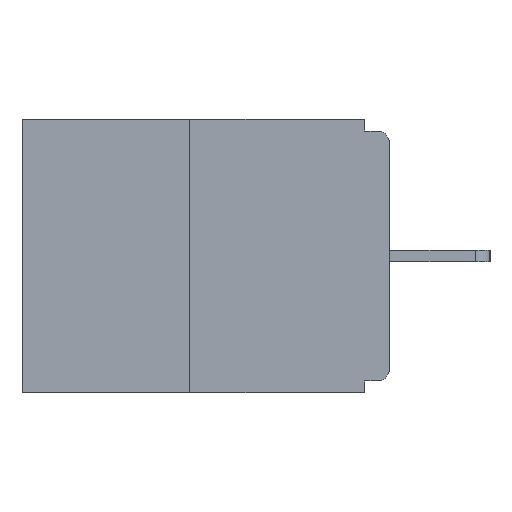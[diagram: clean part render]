
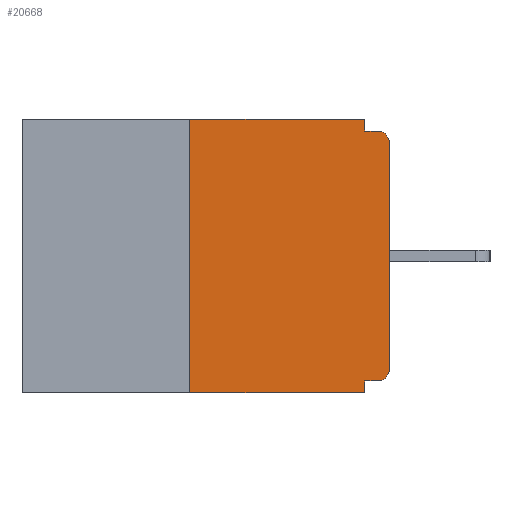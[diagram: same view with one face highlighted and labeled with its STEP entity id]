
A CAD part, left-side view. The second image highlights one B-rep face of the part: STEP entity #20668.
In plain terms, the highlighted planar face has unit normal (-1, 0, 0).
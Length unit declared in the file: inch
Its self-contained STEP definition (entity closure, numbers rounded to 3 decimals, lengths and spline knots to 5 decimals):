
#95 = EDGE_CURVE ( 'NONE', #3770, #21573, #4063, .T. ) ;
#250 = CARTESIAN_POINT ( 'NONE',  ( 0., 0.031, 0. ) ) ;
#340 = VECTOR ( 'NONE', #15545, 39.37008 ) ;
#508 = CARTESIAN_POINT ( 'NONE',  ( 0., 0.031, 0. ) ) ;
#1154 = VERTEX_POINT ( 'NONE', #3916 ) ;
#1259 = DIRECTION ( 'NONE',  ( -1., 0., 0. ) ) ;
#1460 = CARTESIAN_POINT ( 'NONE',  ( 0., 0.015, -0.328 ) ) ;
#1532 = EDGE_CURVE ( 'NONE', #21573, #20040, #19055, .T. ) ;
#1893 = DIRECTION ( 'NONE',  ( 0., -1., 0. ) ) ;
#2144 = DIRECTION ( 'NONE',  ( 0., 0., -1. ) ) ;
#2250 = ORIENTED_EDGE ( 'NONE', *, *, #19633, .T. ) ;
#2343 = CARTESIAN_POINT ( 'NONE',  ( 0., 0.25, 0. ) ) ;
#2382 = EDGE_CURVE ( 'NONE', #19402, #3770, #9972, .T. ) ;
#3080 = LINE ( 'NONE', #21644, #3811 ) ;
#3449 = LINE ( 'NONE', #3668, #11218 ) ;
#3616 = LINE ( 'NONE', #8801, #340 ) ;
#3668 = CARTESIAN_POINT ( 'NONE',  ( 0., 0.46, -0.343 ) ) ;
#3770 = VERTEX_POINT ( 'NONE', #19185 ) ;
#3811 = VECTOR ( 'NONE', #6506, 39.37008 ) ;
#3837 = LINE ( 'NONE', #508, #6637 ) ;
#3916 = CARTESIAN_POINT ( 'NONE',  ( 0., 0.031, -0.015 ) ) ;
#3955 = DIRECTION ( 'NONE',  ( 0., 0., 1. ) ) ;
#4018 = ORIENTED_EDGE ( 'NONE', *, *, #1532, .T. ) ;
#4038 = EDGE_CURVE ( 'NONE', #14052, #16730, #12008, .T. ) ;
#4063 = LINE ( 'NONE', #20645, #6922 ) ;
#4556 = ORIENTED_EDGE ( 'NONE', *, *, #2382, .T. ) ;
#5302 = AXIS2_PLACEMENT_3D ( 'NONE', #16389, #1259, #7968 ) ;
#5350 = PLANE ( 'NONE',  #6602 ) ;
#5366 = DIRECTION ( 'NONE',  ( 0., 0., 1. ) ) ;
#5571 = VECTOR ( 'NONE', #16714, 39.37008 ) ;
#5863 = VERTEX_POINT ( 'NONE', #250 ) ;
#5922 = VECTOR ( 'NONE', #5366, 39.37008 ) ;
#6506 = DIRECTION ( 'NONE',  ( 0., -1., 0. ) ) ;
#6602 = AXIS2_PLACEMENT_3D ( 'NONE', #15522, #11878, #2144 ) ;
#6626 = ORIENTED_EDGE ( 'NONE', *, *, #11526, .F. ) ;
#6637 = VECTOR ( 'NONE', #8999, 39.37008 ) ;
#6922 = VECTOR ( 'NONE', #3955, 39.37008 ) ;
#7847 = DIRECTION ( 'NONE',  ( 0., 0., -1. ) ) ;
#7968 = DIRECTION ( 'NONE',  ( 0., 0., -1. ) ) ;
#8144 = DIRECTION ( 'NONE',  ( 0., 0., -1. ) ) ;
#8559 = ORIENTED_EDGE ( 'NONE', *, *, #95, .T. ) ;
#8592 = CARTESIAN_POINT ( 'NONE',  ( 0., 0.031, -0.328 ) ) ;
#8801 = CARTESIAN_POINT ( 'NONE',  ( 0., 0., -0.328 ) ) ;
#8980 = FACE_OUTER_BOUND ( 'NONE', #16763, .T. ) ;
#8999 = DIRECTION ( 'NONE',  ( 0., 0., -1. ) ) ;
#9675 = EDGE_CURVE ( 'NONE', #1154, #20040, #3080, .T. ) ;
#9744 = EDGE_CURVE ( 'NONE', #5863, #1154, #3837, .T. ) ;
#9869 = VERTEX_POINT ( 'NONE', #12994 ) ;
#9972 = CIRCLE ( 'NONE', #19124, 0.015 ) ;
#10105 = ORIENTED_EDGE ( 'NONE', *, *, #10378, .F. ) ;
#10378 = EDGE_CURVE ( 'NONE', #13232, #9869, #21122, .T. ) ;
#10907 = CARTESIAN_POINT ( 'NONE',  ( 0., 0., -0.03 ) ) ;
#11218 = VECTOR ( 'NONE', #1893, 39.37008 ) ;
#11261 = CARTESIAN_POINT ( 'NONE',  ( 0., 0.015, -0.313 ) ) ;
#11526 = EDGE_CURVE ( 'NONE', #19402, #13232, #3616, .T. ) ;
#11878 = DIRECTION ( 'NONE',  ( 1., 0., 0. ) ) ;
#12008 = LINE ( 'NONE', #18848, #5922 ) ;
#12994 = CARTESIAN_POINT ( 'NONE',  ( 0., 0.031, -0.343 ) ) ;
#13053 = ORIENTED_EDGE ( 'NONE', *, *, #19624, .F. ) ;
#13232 = VERTEX_POINT ( 'NONE', #8592 ) ;
#13514 = CARTESIAN_POINT ( 'NONE',  ( 0., 0.25, -0.343 ) ) ;
#13737 = LINE ( 'NONE', #17038, #5571 ) ;
#14052 = VERTEX_POINT ( 'NONE', #13514 ) ;
#14295 = ORIENTED_EDGE ( 'NONE', *, *, #9675, .F. ) ;
#15163 = ORIENTED_EDGE ( 'NONE', *, *, #4038, .F. ) ;
#15522 = CARTESIAN_POINT ( 'NONE',  ( 0., 0.46, 0. ) ) ;
#15545 = DIRECTION ( 'NONE',  ( 0., 1., 0. ) ) ;
#16389 = CARTESIAN_POINT ( 'NONE',  ( 0., 0.015, -0.03 ) ) ;
#16714 = DIRECTION ( 'NONE',  ( 0., -1., 0. ) ) ;
#16730 = VERTEX_POINT ( 'NONE', #2343 ) ;
#16763 = EDGE_LOOP ( 'NONE', ( #13053, #15163, #2250, #10105, #6626, #4556, #8559, #4018, #14295, #17769 ) ) ;
#17038 = CARTESIAN_POINT ( 'NONE',  ( 0., 0.46, 0. ) ) ;
#17769 = ORIENTED_EDGE ( 'NONE', *, *, #9744, .F. ) ;
#17994 = DIRECTION ( 'NONE',  ( -1., 0., 0. ) ) ;
#18848 = CARTESIAN_POINT ( 'NONE',  ( 0., 0.25, 0. ) ) ;
#19055 = CIRCLE ( 'NONE', #5302, 0.015 ) ;
#19124 = AXIS2_PLACEMENT_3D ( 'NONE', #11261, #17994, #8144 ) ;
#19185 = CARTESIAN_POINT ( 'NONE',  ( 0., 0., -0.313 ) ) ;
#19402 = VERTEX_POINT ( 'NONE', #1460 ) ;
#19624 = EDGE_CURVE ( 'NONE', #16730, #5863, #13737, .T. ) ;
#19633 = EDGE_CURVE ( 'NONE', #14052, #9869, #3449, .T. ) ;
#20040 = VERTEX_POINT ( 'NONE', #20317 ) ;
#20317 = CARTESIAN_POINT ( 'NONE',  ( 0., 0.015, -0.015 ) ) ;
#20645 = CARTESIAN_POINT ( 'NONE',  ( 0., 0., 0. ) ) ;
#20668 = ADVANCED_FACE ( 'NONE', ( #8980 ), #5350, .F. ) ;
#21122 = LINE ( 'NONE', #21231, #21189 ) ;
#21189 = VECTOR ( 'NONE', #7847, 39.37008 ) ;
#21231 = CARTESIAN_POINT ( 'NONE',  ( 0., 0.031, -0.343 ) ) ;
#21573 = VERTEX_POINT ( 'NONE', #10907 ) ;
#21644 = CARTESIAN_POINT ( 'NONE',  ( 0., 0., -0.015 ) ) ;
